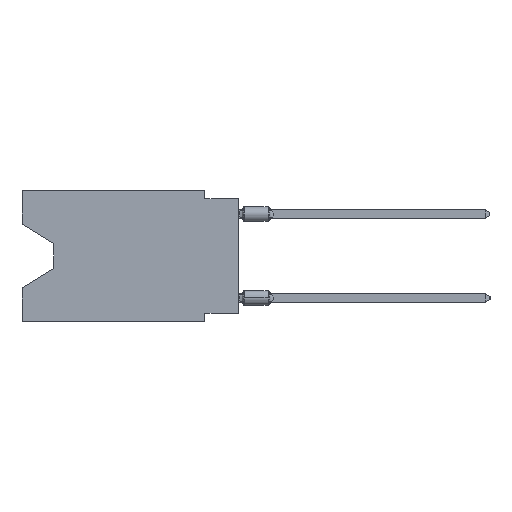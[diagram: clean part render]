
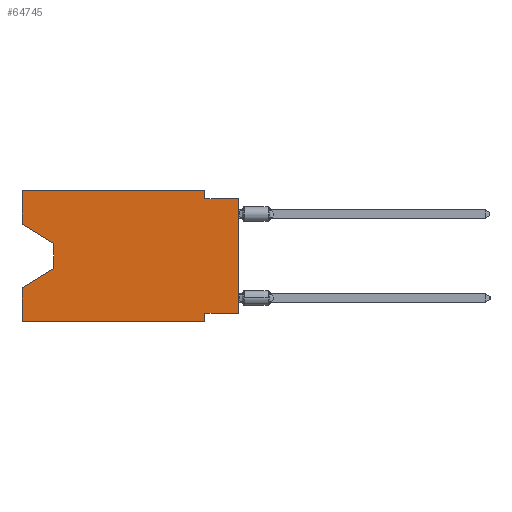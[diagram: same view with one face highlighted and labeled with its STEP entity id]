
A CAD part, left-side view. The second image highlights one B-rep face of the part: STEP entity #64745.
In plain terms, the highlighted planar face has unit normal (-1, 0, 0).
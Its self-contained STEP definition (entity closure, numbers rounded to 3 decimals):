
#970 = CARTESIAN_POINT ( 'NONE',  ( 0., 16.383, -2.546 ) ) ;
#1709 = ORIENTED_EDGE ( 'NONE', *, *, #17916, .F. ) ;
#4148 = ORIENTED_EDGE ( 'NONE', *, *, #13146, .F. ) ;
#4375 = VERTEX_POINT ( 'NONE', #31687 ) ;
#5182 = VERTEX_POINT ( 'NONE', #57113 ) ;
#5382 = ORIENTED_EDGE ( 'NONE', *, *, #10298, .T. ) ;
#5579 = LINE ( 'NONE', #970, #29681 ) ;
#7576 = VECTOR ( 'NONE', #22402, 1000. ) ;
#8149 = DIRECTION ( 'NONE',  ( 0., -1., 0. ) ) ;
#8960 = CARTESIAN_POINT ( 'NONE',  ( 0., 0., -0.635 ) ) ;
#9324 = VECTOR ( 'NONE', #14724, 1000. ) ;
#9800 = LINE ( 'NONE', #38994, #9324 ) ;
#10298 = EDGE_CURVE ( 'NONE', #53931, #56342, #21967, .T. ) ;
#11099 = VECTOR ( 'NONE', #33895, 1000. ) ;
#11161 = LINE ( 'NONE', #30536, #30757 ) ;
#12314 = CARTESIAN_POINT ( 'NONE',  ( 0., 2.54, 0. ) ) ;
#12878 = LINE ( 'NONE', #47971, #63812 ) ;
#13146 = EDGE_CURVE ( 'NONE', #19954, #5182, #22340, .T. ) ;
#13194 = DIRECTION ( 'NONE',  ( 0., 0., 1. ) ) ;
#13215 = VERTEX_POINT ( 'NONE', #60337 ) ;
#14533 = VECTOR ( 'NONE', #18729, 1000. ) ;
#14570 = VECTOR ( 'NONE', #40287, 1000. ) ;
#14724 = DIRECTION ( 'NONE',  ( 0., 0., -1. ) ) ;
#16089 = DIRECTION ( 'NONE',  ( 0., 0., 1. ) ) ;
#16211 = VERTEX_POINT ( 'NONE', #21746 ) ;
#16216 = ORIENTED_EDGE ( 'NONE', *, *, #60565, .T. ) ;
#17093 = VERTEX_POINT ( 'NONE', #12314 ) ;
#17153 = LINE ( 'NONE', #32233, #7576 ) ;
#17313 = CARTESIAN_POINT ( 'NONE',  ( 0., 2.54, -9.906 ) ) ;
#17916 = EDGE_CURVE ( 'NONE', #17093, #24303, #42638, .T. ) ;
#18358 = EDGE_LOOP ( 'NONE', ( #64808, #55766, #5382, #60085, #16216, #33116, #4148, #44032, #21968, #1709, #53092, #22685 ) ) ;
#18729 = DIRECTION ( 'NONE',  ( 0., 1., 0. ) ) ;
#19539 = EDGE_CURVE ( 'NONE', #4375, #17093, #17153, .T. ) ;
#19954 = VERTEX_POINT ( 'NONE', #36417 ) ;
#20825 = PLANE ( 'NONE',  #39591 ) ;
#20940 = LINE ( 'NONE', #45219, #14570 ) ;
#21746 = CARTESIAN_POINT ( 'NONE',  ( 0., 16.383, -2.546 ) ) ;
#21967 = LINE ( 'NONE', #50850, #54417 ) ;
#21968 = ORIENTED_EDGE ( 'NONE', *, *, #33512, .F. ) ;
#22340 = LINE ( 'NONE', #42334, #14533 ) ;
#22402 = DIRECTION ( 'NONE',  ( 0., -1., 0. ) ) ;
#22488 = CARTESIAN_POINT ( 'NONE',  ( 0., 2.54, -0.635 ) ) ;
#22604 = LINE ( 'NONE', #42599, #41506 ) ;
#22685 = ORIENTED_EDGE ( 'NONE', *, *, #42101, .F. ) ;
#23992 = VERTEX_POINT ( 'NONE', #17313 ) ;
#24303 = VERTEX_POINT ( 'NONE', #22488 ) ;
#28531 = CARTESIAN_POINT ( 'NONE',  ( 0., 16.383, -9.906 ) ) ;
#29681 = VECTOR ( 'NONE', #50517, 1000. ) ;
#30139 = CARTESIAN_POINT ( 'NONE',  ( 0., 13.97, -5.893 ) ) ;
#30342 = DIRECTION ( 'NONE',  ( 0., 0., -1. ) ) ;
#30536 = CARTESIAN_POINT ( 'NONE',  ( 0., 16.383, 0. ) ) ;
#30757 = VECTOR ( 'NONE', #16089, 1000. ) ;
#31687 = CARTESIAN_POINT ( 'NONE',  ( 0., 16.383, 0. ) ) ;
#32233 = CARTESIAN_POINT ( 'NONE',  ( 0., 16.383, 0. ) ) ;
#33116 = ORIENTED_EDGE ( 'NONE', *, *, #48775, .F. ) ;
#33512 = EDGE_CURVE ( 'NONE', #24303, #13215, #33568, .T. ) ;
#33568 = LINE ( 'NONE', #8960, #11099 ) ;
#33895 = DIRECTION ( 'NONE',  ( 0., -1., 0. ) ) ;
#34840 = VECTOR ( 'NONE', #36756, 1000. ) ;
#36417 = CARTESIAN_POINT ( 'NONE',  ( 0., 0., -9.271 ) ) ;
#36756 = DIRECTION ( 'NONE',  ( 0., 0., -1. ) ) ;
#37980 = EDGE_CURVE ( 'NONE', #19954, #13215, #12878, .T. ) ;
#38636 = VERTEX_POINT ( 'NONE', #28531 ) ;
#38994 = CARTESIAN_POINT ( 'NONE',  ( 0., 2.54, -9.906 ) ) ;
#39591 = AXIS2_PLACEMENT_3D ( 'NONE', #45423, #51316, #30342 ) ;
#40287 = DIRECTION ( 'NONE',  ( 0., 0., 1. ) ) ;
#41472 = CARTESIAN_POINT ( 'NONE',  ( 0., 13.97, -4.013 ) ) ;
#41506 = VECTOR ( 'NONE', #8149, 1000. ) ;
#41665 = CARTESIAN_POINT ( 'NONE',  ( 0., 2.54, 0. ) ) ;
#42101 = EDGE_CURVE ( 'NONE', #16211, #4375, #11161, .T. ) ;
#42334 = CARTESIAN_POINT ( 'NONE',  ( 0., 0., -9.271 ) ) ;
#42599 = CARTESIAN_POINT ( 'NONE',  ( 0., 16.383, -9.906 ) ) ;
#42638 = LINE ( 'NONE', #41665, #34840 ) ;
#43344 = EDGE_CURVE ( 'NONE', #16211, #48249, #5579, .T. ) ;
#44032 = ORIENTED_EDGE ( 'NONE', *, *, #37980, .T. ) ;
#44056 = CARTESIAN_POINT ( 'NONE',  ( 0., 13.97, -4.013 ) ) ;
#45219 = CARTESIAN_POINT ( 'NONE',  ( 0., 16.383, 0. ) ) ;
#45423 = CARTESIAN_POINT ( 'NONE',  ( 0., 16.383, 0. ) ) ;
#45921 = DIRECTION ( 'NONE',  ( 0., 0.855, -0.519 ) ) ;
#47971 = CARTESIAN_POINT ( 'NONE',  ( 0., 0., 0. ) ) ;
#48249 = VERTEX_POINT ( 'NONE', #41472 ) ;
#48775 = EDGE_CURVE ( 'NONE', #5182, #23992, #9800, .T. ) ;
#48895 = EDGE_CURVE ( 'NONE', #38636, #56342, #20940, .T. ) ;
#49291 = DIRECTION ( 'NONE',  ( 0., 0., -1. ) ) ;
#50517 = DIRECTION ( 'NONE',  ( 0., -0.855, -0.519 ) ) ;
#50850 = CARTESIAN_POINT ( 'NONE',  ( 0., 13.97, -5.893 ) ) ;
#51316 = DIRECTION ( 'NONE',  ( 1., 0., 0. ) ) ;
#53092 = ORIENTED_EDGE ( 'NONE', *, *, #19539, .F. ) ;
#53931 = VERTEX_POINT ( 'NONE', #30139 ) ;
#54220 = LINE ( 'NONE', #44056, #57315 ) ;
#54417 = VECTOR ( 'NONE', #45921, 1000. ) ;
#55766 = ORIENTED_EDGE ( 'NONE', *, *, #63734, .T. ) ;
#56342 = VERTEX_POINT ( 'NONE', #64534 ) ;
#57113 = CARTESIAN_POINT ( 'NONE',  ( 0., 2.54, -9.271 ) ) ;
#57315 = VECTOR ( 'NONE', #49291, 1000. ) ;
#60085 = ORIENTED_EDGE ( 'NONE', *, *, #48895, .F. ) ;
#60197 = FACE_OUTER_BOUND ( 'NONE', #18358, .T. ) ;
#60337 = CARTESIAN_POINT ( 'NONE',  ( 0., 0., -0.635 ) ) ;
#60565 = EDGE_CURVE ( 'NONE', #38636, #23992, #22604, .T. ) ;
#63734 = EDGE_CURVE ( 'NONE', #48249, #53931, #54220, .T. ) ;
#63812 = VECTOR ( 'NONE', #13194, 1000. ) ;
#64534 = CARTESIAN_POINT ( 'NONE',  ( 0., 16.383, -7.36 ) ) ;
#64745 = ADVANCED_FACE ( 'NONE', ( #60197 ), #20825, .F. ) ;
#64808 = ORIENTED_EDGE ( 'NONE', *, *, #43344, .T. ) ;
